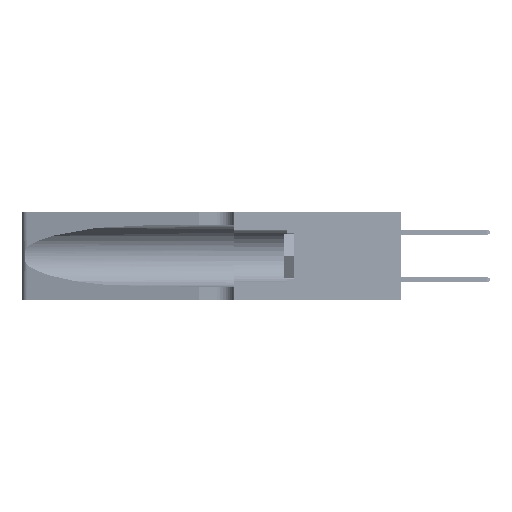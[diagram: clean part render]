
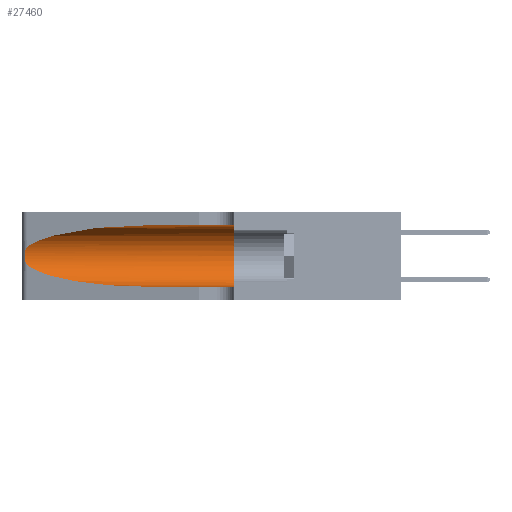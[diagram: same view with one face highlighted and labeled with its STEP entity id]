
A CAD part, left-side view. The second image highlights one B-rep face of the part: STEP entity #27460.
In plain terms, the highlighted cylindrical face has radius 3.308 mm (diameter 6.617 mm), a partial arc.
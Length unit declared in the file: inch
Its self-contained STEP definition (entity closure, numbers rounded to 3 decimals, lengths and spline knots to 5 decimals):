
#562 = CARTESIAN_POINT ( 'NONE',  ( 0.26075, 1.23896, 0.19203 ) ) ;
#747 = CARTESIAN_POINT ( 'NONE',  ( 0.25555, 1.22994, 0.2215 ) ) ;
#770 = DIRECTION ( 'NONE',  ( 0., -1., 0. ) ) ;
#2474 = LINE ( 'NONE', #12636, #20403 ) ;
#3126 = VECTOR ( 'NONE', #770, 39.37008 ) ;
#3915 = ORIENTED_EDGE ( 'NONE', *, *, #43833, .T. ) ;
#4512 = CARTESIAN_POINT ( 'NONE',  ( 0.25789, 1.23486, 0.15765 ) ) ;
#5693 = LINE ( 'NONE', #25221, #3126 ) ;
#6048 = CARTESIAN_POINT ( 'NONE',  ( 0.1305, 0.35, 0.31525 ) ) ;
#6322 =( BOUNDED_CURVE ( )  B_SPLINE_CURVE ( 3, ( #29357, #29698, #37704, #8836 ),
 .UNSPECIFIED., .F., .F. ) 
 B_SPLINE_CURVE_WITH_KNOTS ( ( 4, 4 ),
 ( 3.44316, 4.71239 ),
 .UNSPECIFIED. ) 
 CURVE ( )  GEOMETRIC_REPRESENTATION_ITEM ( )  RATIONAL_B_SPLINE_CURVE ( ( 1., 0.87, 0.87, 1. ) ) 
 REPRESENTATION_ITEM ( '' )  );
#8458 = CARTESIAN_POINT ( 'NONE',  ( 0.26018, 1.23835, 0.19895 ) ) ;
#8638 = CARTESIAN_POINT ( 'NONE',  ( 0.25639, 1.23186, 0.15144 ) ) ;
#8836 = CARTESIAN_POINT ( 'NONE',  ( 0.1305, 0.72297, 0.05475 ) ) ;
#8961 = DIRECTION ( 'NONE',  ( 0., -1., 0. ) ) ;
#11540 = CARTESIAN_POINT ( 'NONE',  ( 0.1305, 0.72297, 0.31525 ) ) ;
#12636 = CARTESIAN_POINT ( 'NONE',  ( 0.1305, 1.61858, 0.31525 ) ) ;
#13444 = EDGE_CURVE ( 'NONE', #16550, #20589, #2474, .T. ) ;
#13643 = CARTESIAN_POINT ( 'NONE',  ( 0.1305, 0.35, 0.185 ) ) ;
#16370 = AXIS2_PLACEMENT_3D ( 'NONE', #13643, #33782, #42170 ) ;
#16550 = VERTEX_POINT ( 'NONE', #11540 ) ;
#16673 = CARTESIAN_POINT ( 'NONE',  ( 0.26075, 1.23896, 0.178 ) ) ;
#17363 = CARTESIAN_POINT ( 'NONE',  ( 0.1305, 1.61858, 0.185 ) ) ;
#18299 = EDGE_LOOP ( 'NONE', ( #3915, #52183, #34299, #35740, #24377, #51930 ) ) ;
#20403 = VECTOR ( 'NONE', #36542, 39.37008 ) ;
#20589 = VERTEX_POINT ( 'NONE', #6048 ) ;
#22234 = VERTEX_POINT ( 'NONE', #45771 ) ;
#24377 = ORIENTED_EDGE ( 'NONE', *, *, #27982, .F. ) ;
#24688 = CARTESIAN_POINT ( 'NONE',  ( 0.25487, 1.22718, 0.22369 ) ) ;
#24862 = CARTESIAN_POINT ( 'NONE',  ( 0.26017, 1.23833, 0.17102 ) ) ;
#25221 = CARTESIAN_POINT ( 'NONE',  ( 0.1305, 1.61858, 0.05475 ) ) ;
#25275 = B_SPLINE_CURVE_WITH_KNOTS ( 'NONE', 3,
 ( #24688, #747, #33375, #28784, #32854, #8458, #562, #16673, #24862, #28956, #4512, #8638, #37132, #49459 ),
 .UNSPECIFIED., .F., .F.,
 ( 4, 2, 2, 2, 2, 2, 4 ),
 ( 0., 0.00027, 0.00053, 0.00107, 0.0016, 0.00187, 0.00214 ),
 .UNSPECIFIED. ) ;
#27460 = ADVANCED_FACE ( 'NONE', ( #41750 ), #34077, .F. ) ;
#27829 = VERTEX_POINT ( 'NONE', #49860 ) ;
#27883 =( BOUNDED_CURVE ( )  B_SPLINE_CURVE ( 3, ( #42136, #49997, #38194, #29844 ),
 .UNSPECIFIED., .F., .F. ) 
 B_SPLINE_CURVE_WITH_KNOTS ( ( 4, 4 ),
 ( 1.5708, 2.84003 ),
 .UNSPECIFIED. ) 
 CURVE ( )  GEOMETRIC_REPRESENTATION_ITEM ( )  RATIONAL_B_SPLINE_CURVE ( ( 1., 0.87, 0.87, 1. ) ) 
 REPRESENTATION_ITEM ( '' )  );
#27982 = EDGE_CURVE ( 'NONE', #20589, #22234, #46878, .T. ) ;
#28615 = AXIS2_PLACEMENT_3D ( 'NONE', #17363, #8961, #37466 ) ;
#28784 = CARTESIAN_POINT ( 'NONE',  ( 0.25787, 1.23484, 0.2124 ) ) ;
#28956 = CARTESIAN_POINT ( 'NONE',  ( 0.25856, 1.23593, 0.16098 ) ) ;
#29357 = CARTESIAN_POINT ( 'NONE',  ( 0.25487, 1.22718, 0.14631 ) ) ;
#29698 = CARTESIAN_POINT ( 'NONE',  ( 0.2373, 1.15595, 0.08982 ) ) ;
#29844 = CARTESIAN_POINT ( 'NONE',  ( 0.25487, 1.22718, 0.22369 ) ) ;
#31542 = VERTEX_POINT ( 'NONE', #37167 ) ;
#32854 = CARTESIAN_POINT ( 'NONE',  ( 0.25854, 1.2359, 0.20912 ) ) ;
#33375 = CARTESIAN_POINT ( 'NONE',  ( 0.25639, 1.23184, 0.21858 ) ) ;
#33782 = DIRECTION ( 'NONE',  ( 0., 1., 0. ) ) ;
#34077 = CYLINDRICAL_SURFACE ( 'NONE', #28615, 0.13025 ) ;
#34299 = ORIENTED_EDGE ( 'NONE', *, *, #47324, .T. ) ;
#35740 = ORIENTED_EDGE ( 'NONE', *, *, #40319, .T. ) ;
#36542 = DIRECTION ( 'NONE',  ( 0., -1., 0. ) ) ;
#37132 = CARTESIAN_POINT ( 'NONE',  ( 0.25555, 1.22993, 0.14849 ) ) ;
#37167 = CARTESIAN_POINT ( 'NONE',  ( 0.1305, 0.72297, 0.05475 ) ) ;
#37466 = DIRECTION ( 'NONE',  ( 0., 0., -1. ) ) ;
#37704 = CARTESIAN_POINT ( 'NONE',  ( 0.18966, 0.96281, 0.05475 ) ) ;
#38194 = CARTESIAN_POINT ( 'NONE',  ( 0.2373, 1.15595, 0.28018 ) ) ;
#38962 = EDGE_CURVE ( 'NONE', #27829, #48353, #25275, .T. ) ;
#40319 = EDGE_CURVE ( 'NONE', #31542, #22234, #5693, .T. ) ;
#41750 = FACE_OUTER_BOUND ( 'NONE', #18299, .T. ) ;
#42136 = CARTESIAN_POINT ( 'NONE',  ( 0.1305, 0.72297, 0.31525 ) ) ;
#42170 = DIRECTION ( 'NONE',  ( 0., 0., 1. ) ) ;
#43833 = EDGE_CURVE ( 'NONE', #16550, #27829, #27883, .T. ) ;
#45771 = CARTESIAN_POINT ( 'NONE',  ( 0.1305, 0.35, 0.05475 ) ) ;
#46878 = CIRCLE ( 'NONE', #16370, 0.13025 ) ;
#47324 = EDGE_CURVE ( 'NONE', #48353, #31542, #6322, .T. ) ;
#48353 = VERTEX_POINT ( 'NONE', #48687 ) ;
#48687 = CARTESIAN_POINT ( 'NONE',  ( 0.25487, 1.22718, 0.14631 ) ) ;
#49459 = CARTESIAN_POINT ( 'NONE',  ( 0.25487, 1.22718, 0.14631 ) ) ;
#49860 = CARTESIAN_POINT ( 'NONE',  ( 0.25487, 1.22718, 0.22369 ) ) ;
#49997 = CARTESIAN_POINT ( 'NONE',  ( 0.18966, 0.96281, 0.31525 ) ) ;
#51930 = ORIENTED_EDGE ( 'NONE', *, *, #13444, .F. ) ;
#52183 = ORIENTED_EDGE ( 'NONE', *, *, #38962, .T. ) ;
